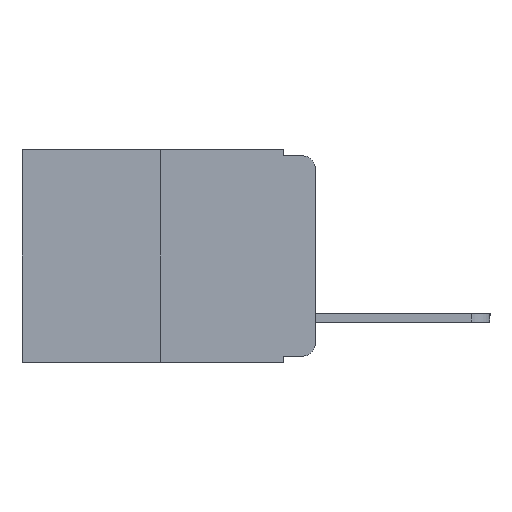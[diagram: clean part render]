
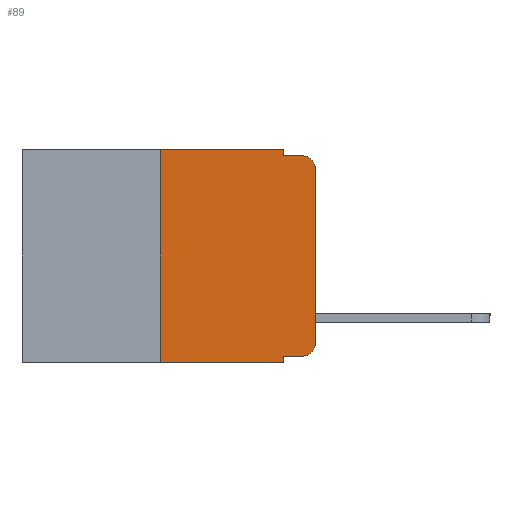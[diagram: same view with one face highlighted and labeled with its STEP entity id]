
A CAD part, left-side view. The second image highlights one B-rep face of the part: STEP entity #89.
In plain terms, the highlighted planar face has unit normal (-1, 0, 0).
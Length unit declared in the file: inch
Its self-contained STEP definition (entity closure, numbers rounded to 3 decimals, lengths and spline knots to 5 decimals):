
#38 = CARTESIAN_POINT ( 'NONE',  ( 0., 0.051, -0.333 ) ) ;
#45 = DIRECTION ( 'NONE',  ( 0., 0., 1. ) ) ;
#89 = ADVANCED_FACE ( 'NONE', ( #7472 ), #6176, .F. ) ;
#121 = LINE ( 'NONE', #8085, #3571 ) ;
#176 = VECTOR ( 'NONE', #15369, 39.37008 ) ;
#214 = ORIENTED_EDGE ( 'NONE', *, *, #739, .F. ) ;
#252 = LINE ( 'NONE', #14080, #3294 ) ;
#377 = DIRECTION ( 'NONE',  ( 0., -1., 0. ) ) ;
#645 = ORIENTED_EDGE ( 'NONE', *, *, #15515, .F. ) ;
#678 = CARTESIAN_POINT ( 'NONE',  ( 0., 0.051, -0.333 ) ) ;
#739 = EDGE_CURVE ( 'NONE', #8531, #1415, #13799, .T. ) ;
#1064 = ORIENTED_EDGE ( 'NONE', *, *, #14703, .F. ) ;
#1174 = DIRECTION ( 'NONE',  ( -1., 0., 0. ) ) ;
#1415 = VERTEX_POINT ( 'NONE', #10617 ) ;
#1433 = CARTESIAN_POINT ( 'NONE',  ( 0., 0.051, 0. ) ) ;
#1589 = EDGE_CURVE ( 'NONE', #1415, #10752, #4407, .T. ) ;
#1834 = AXIS2_PLACEMENT_3D ( 'NONE', #13070, #5419, #14288 ) ;
#1964 = DIRECTION ( 'NONE',  ( 0., 0., -1. ) ) ;
#2491 = VECTOR ( 'NONE', #8062, 39.37008 ) ;
#2579 = EDGE_CURVE ( 'NONE', #5714, #8531, #121, .T. ) ;
#2584 = CIRCLE ( 'NONE', #12050, 0.02 ) ;
#3041 = CARTESIAN_POINT ( 'NONE',  ( 0., 0.473, -0.343 ) ) ;
#3262 = ORIENTED_EDGE ( 'NONE', *, *, #3323, .T. ) ;
#3294 = VECTOR ( 'NONE', #45, 39.37008 ) ;
#3323 = EDGE_CURVE ( 'NONE', #9519, #10752, #2584, .T. ) ;
#3571 = VECTOR ( 'NONE', #377, 39.37008 ) ;
#3572 = LINE ( 'NONE', #9751, #10892 ) ;
#3695 = CARTESIAN_POINT ( 'NONE',  ( 0., 0.051, -0.343 ) ) ;
#3895 = VECTOR ( 'NONE', #8251, 39.37008 ) ;
#4222 = CARTESIAN_POINT ( 'NONE',  ( 0., 0., 0. ) ) ;
#4407 = LINE ( 'NONE', #16218, #10518 ) ;
#4531 = VERTEX_POINT ( 'NONE', #38 ) ;
#4684 = CARTESIAN_POINT ( 'NONE',  ( 0., 0.02, -0.03 ) ) ;
#5419 = DIRECTION ( 'NONE',  ( -1., 0., 0. ) ) ;
#5714 = VERTEX_POINT ( 'NONE', #15174 ) ;
#5918 = CARTESIAN_POINT ( 'NONE',  ( 0., 0.25, -0.343 ) ) ;
#5933 = CARTESIAN_POINT ( 'NONE',  ( 0., 0., -0.03 ) ) ;
#5943 = EDGE_CURVE ( 'NONE', #15732, #9519, #9412, .T. ) ;
#6176 = PLANE ( 'NONE',  #12925 ) ;
#6237 = CARTESIAN_POINT ( 'NONE',  ( 0., 0.02, -0.01 ) ) ;
#6380 = CARTESIAN_POINT ( 'NONE',  ( 0., 0.051, 0. ) ) ;
#6668 = DIRECTION ( 'NONE',  ( 0., 0., -1. ) ) ;
#6720 = ORIENTED_EDGE ( 'NONE', *, *, #1589, .F. ) ;
#6722 = LINE ( 'NONE', #678, #8953 ) ;
#6904 = EDGE_LOOP ( 'NONE', ( #9791, #3262, #6720, #214, #10581, #645, #10992, #1064, #7910, #14587 ) ) ;
#6946 = LINE ( 'NONE', #3041, #3895 ) ;
#6961 = VERTEX_POINT ( 'NONE', #3695 ) ;
#7472 = FACE_OUTER_BOUND ( 'NONE', #6904, .T. ) ;
#7721 = CARTESIAN_POINT ( 'NONE',  ( 0., 0.02, -0.333 ) ) ;
#7910 = ORIENTED_EDGE ( 'NONE', *, *, #12265, .T. ) ;
#8062 = DIRECTION ( 'NONE',  ( 0., 0., 1. ) ) ;
#8085 = CARTESIAN_POINT ( 'NONE',  ( 0., 0.473, 0. ) ) ;
#8251 = DIRECTION ( 'NONE',  ( 0., -1., 0. ) ) ;
#8531 = VERTEX_POINT ( 'NONE', #1433 ) ;
#8729 = DIRECTION ( 'NONE',  ( 0., -1., 0. ) ) ;
#8951 = CARTESIAN_POINT ( 'NONE',  ( 0., 0.473, 0. ) ) ;
#8953 = VECTOR ( 'NONE', #14692, 39.37008 ) ;
#9114 = DIRECTION ( 'NONE',  ( 1., 0., 0. ) ) ;
#9408 = CIRCLE ( 'NONE', #1834, 0.02 ) ;
#9412 = LINE ( 'NONE', #4222, #2491 ) ;
#9519 = VERTEX_POINT ( 'NONE', #5933 ) ;
#9751 = CARTESIAN_POINT ( 'NONE',  ( 0., 0.051, 0. ) ) ;
#9791 = ORIENTED_EDGE ( 'NONE', *, *, #5943, .T. ) ;
#10518 = VECTOR ( 'NONE', #8729, 39.37008 ) ;
#10581 = ORIENTED_EDGE ( 'NONE', *, *, #2579, .F. ) ;
#10617 = CARTESIAN_POINT ( 'NONE',  ( 0., 0.051, -0.01 ) ) ;
#10752 = VERTEX_POINT ( 'NONE', #6237 ) ;
#10884 = CARTESIAN_POINT ( 'NONE',  ( 0., 0., -0.313 ) ) ;
#10892 = VECTOR ( 'NONE', #1964, 39.37008 ) ;
#10992 = ORIENTED_EDGE ( 'NONE', *, *, #15717, .T. ) ;
#11448 = EDGE_CURVE ( 'NONE', #16079, #15732, #9408, .T. ) ;
#12050 = AXIS2_PLACEMENT_3D ( 'NONE', #4684, #1174, #12471 ) ;
#12265 = EDGE_CURVE ( 'NONE', #4531, #16079, #6722, .T. ) ;
#12471 = DIRECTION ( 'NONE',  ( 0., 0., -1. ) ) ;
#12925 = AXIS2_PLACEMENT_3D ( 'NONE', #8951, #9114, #6668 ) ;
#13070 = CARTESIAN_POINT ( 'NONE',  ( 0., 0.02, -0.313 ) ) ;
#13799 = LINE ( 'NONE', #6380, #176 ) ;
#14080 = CARTESIAN_POINT ( 'NONE',  ( 0., 0.25, 0. ) ) ;
#14288 = DIRECTION ( 'NONE',  ( 0., 0., -1. ) ) ;
#14587 = ORIENTED_EDGE ( 'NONE', *, *, #11448, .T. ) ;
#14692 = DIRECTION ( 'NONE',  ( 0., -1., 0. ) ) ;
#14703 = EDGE_CURVE ( 'NONE', #4531, #6961, #3572, .T. ) ;
#14761 = VERTEX_POINT ( 'NONE', #5918 ) ;
#15174 = CARTESIAN_POINT ( 'NONE',  ( 0., 0.25, 0. ) ) ;
#15369 = DIRECTION ( 'NONE',  ( 0., 0., -1. ) ) ;
#15515 = EDGE_CURVE ( 'NONE', #14761, #5714, #252, .T. ) ;
#15717 = EDGE_CURVE ( 'NONE', #14761, #6961, #6946, .T. ) ;
#15732 = VERTEX_POINT ( 'NONE', #10884 ) ;
#16079 = VERTEX_POINT ( 'NONE', #7721 ) ;
#16218 = CARTESIAN_POINT ( 'NONE',  ( 0., 0.051, -0.01 ) ) ;
